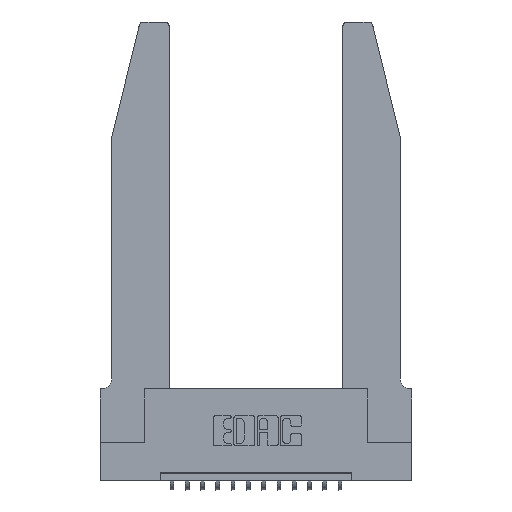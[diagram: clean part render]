
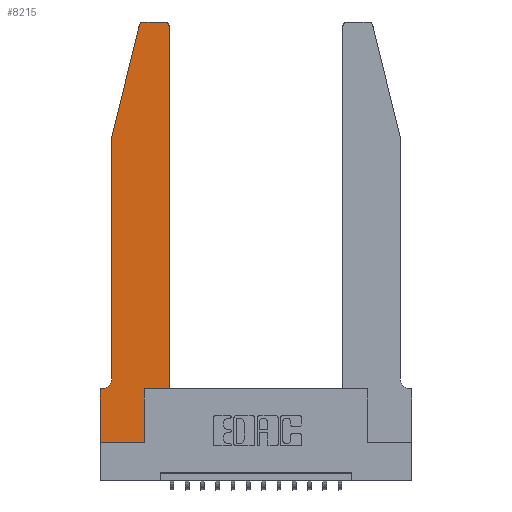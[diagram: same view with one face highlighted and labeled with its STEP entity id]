
A CAD part, top view. The second image highlights one B-rep face of the part: STEP entity #8215.
In plain terms, the highlighted planar face has unit normal (0, 0, 1).
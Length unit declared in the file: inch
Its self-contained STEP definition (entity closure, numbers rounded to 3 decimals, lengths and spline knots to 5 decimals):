
#14 = VERTEX_POINT ( 'NONE', #5899 ) ;
#186 = ORIENTED_EDGE ( 'NONE', *, *, #17065, .T. ) ;
#826 = ORIENTED_EDGE ( 'NONE', *, *, #7847, .T. ) ;
#1065 = CARTESIAN_POINT ( 'NONE',  ( 0.2605, 2.75, 0.37 ) ) ;
#1076 = EDGE_CURVE ( 'NONE', #7995, #10283, #5129, .T. ) ;
#1280 = CIRCLE ( 'NONE', #4419, 0.07 ) ;
#1588 = VERTEX_POINT ( 'NONE', #16901 ) ;
#1635 = EDGE_CURVE ( 'NONE', #1588, #16401, #10755, .T. ) ;
#1659 = VECTOR ( 'NONE', #11710, 39.37008 ) ;
#2126 = CARTESIAN_POINT ( 'NONE',  ( 0., 0., 0.37 ) ) ;
#2230 = CARTESIAN_POINT ( 'NONE',  ( 0.284, 2.72, 0.37 ) ) ;
#2387 = VERTEX_POINT ( 'NONE', #16513 ) ;
#2408 = DIRECTION ( 'NONE',  ( 0., 1., 0. ) ) ;
#2767 = CARTESIAN_POINT ( 'NONE',  ( 0., 0., 0.37 ) ) ;
#3161 = EDGE_CURVE ( 'NONE', #10283, #14, #5533, .T. ) ;
#3262 = VERTEX_POINT ( 'NONE', #2126 ) ;
#3343 = ORIENTED_EDGE ( 'NONE', *, *, #13811, .T. ) ;
#3395 = VECTOR ( 'NONE', #5492, 39.37008 ) ;
#3405 = ORIENTED_EDGE ( 'NONE', *, *, #16926, .T. ) ;
#3450 = ORIENTED_EDGE ( 'NONE', *, *, #16946, .T. ) ;
#3671 = CARTESIAN_POINT ( 'NONE',  ( 0.2865, 0.35, 0.37 ) ) ;
#3999 = AXIS2_PLACEMENT_3D ( 'NONE', #4732, #17258, #11753 ) ;
#4192 = CARTESIAN_POINT ( 'NONE',  ( 0.25487, 2.72718, 0.37 ) ) ;
#4263 = VECTOR ( 'NONE', #7435, 39.37008 ) ;
#4272 = VERTEX_POINT ( 'NONE', #6718 ) ;
#4382 = ORIENTED_EDGE ( 'NONE', *, *, #3161, .T. ) ;
#4390 = DIRECTION ( 'NONE',  ( 0., -1., 0. ) ) ;
#4419 = AXIS2_PLACEMENT_3D ( 'NONE', #12289, #13267, #4938 ) ;
#4446 = CARTESIAN_POINT ( 'NONE',  ( 0., 0., 0.37 ) ) ;
#4488 = FACE_OUTER_BOUND ( 'NONE', #10776, .T. ) ;
#4732 = CARTESIAN_POINT ( 'NONE',  ( 0.4205, 2.72, 0.37 ) ) ;
#4736 = CARTESIAN_POINT ( 'NONE',  ( 0.0755, 2., 0.37 ) ) ;
#4938 = DIRECTION ( 'NONE',  ( -1., 0., 0. ) ) ;
#5013 = AXIS2_PLACEMENT_3D ( 'NONE', #7494, #8884, #10284 ) ;
#5085 = DIRECTION ( 'NONE',  ( 0., 0., 1. ) ) ;
#5129 = LINE ( 'NONE', #14333, #10101 ) ;
#5200 = LINE ( 'NONE', #4446, #15573 ) ;
#5256 = EDGE_CURVE ( 'NONE', #12129, #7332, #7608, .T. ) ;
#5405 = CARTESIAN_POINT ( 'NONE',  ( 0., 0.35, 0.37 ) ) ;
#5492 = DIRECTION ( 'NONE',  ( 1., 0., 0. ) ) ;
#5533 = LINE ( 'NONE', #17791, #8347 ) ;
#5899 = CARTESIAN_POINT ( 'NONE',  ( 0.4505, 2.72, 0.37 ) ) ;
#5978 = LINE ( 'NONE', #1065, #13170 ) ;
#6718 = CARTESIAN_POINT ( 'NONE',  ( 0.2865, 0., 0.37 ) ) ;
#7332 = VERTEX_POINT ( 'NONE', #4736 ) ;
#7435 = DIRECTION ( 'NONE',  ( -1., 0., 0. ) ) ;
#7494 = CARTESIAN_POINT ( 'NONE',  ( 0., 0.35, 0.37 ) ) ;
#7582 = DIRECTION ( 'NONE',  ( 1., 0., 0. ) ) ;
#7608 = LINE ( 'NONE', #14395, #14089 ) ;
#7847 = EDGE_CURVE ( 'NONE', #7332, #11194, #17225, .T. ) ;
#7856 = DIRECTION ( 'NONE',  ( 1., 0., 0. ) ) ;
#7995 = VERTEX_POINT ( 'NONE', #16257 ) ;
#8129 = LINE ( 'NONE', #3671, #8779 ) ;
#8215 = ADVANCED_FACE ( 'NONE', ( #4488 ), #15583, .T. ) ;
#8347 = VECTOR ( 'NONE', #2408, 39.37008 ) ;
#8361 = CIRCLE ( 'NONE', #3999, 0.03 ) ;
#8779 = VECTOR ( 'NONE', #13556, 39.37008 ) ;
#8884 = DIRECTION ( 'NONE',  ( 0., 0., 1. ) ) ;
#8966 = DIRECTION ( 'NONE',  ( -0.239, -0.971, 0. ) ) ;
#9866 = EDGE_CURVE ( 'NONE', #14, #13092, #8361, .T. ) ;
#10101 = VECTOR ( 'NONE', #7582, 39.37008 ) ;
#10283 = VERTEX_POINT ( 'NONE', #16583 ) ;
#10284 = DIRECTION ( 'NONE',  ( 1., 0., 0. ) ) ;
#10676 = EDGE_CURVE ( 'NONE', #4272, #7995, #8129, .T. ) ;
#10755 = LINE ( 'NONE', #11514, #4263 ) ;
#10776 = EDGE_LOOP ( 'NONE', ( #3405, #3450, #16666, #826, #16829, #14975, #3343, #186, #14225, #11814, #4382, #16773 ) ) ;
#11194 = VERTEX_POINT ( 'NONE', #15000 ) ;
#11464 = CARTESIAN_POINT ( 'NONE',  ( 0.0755, 2., 0.37 ) ) ;
#11514 = CARTESIAN_POINT ( 'NONE',  ( 0.0755, 0.35, 0.37 ) ) ;
#11710 = DIRECTION ( 'NONE',  ( 0., -1., 0. ) ) ;
#11753 = DIRECTION ( 'NONE',  ( 1., 0., 0. ) ) ;
#11814 = ORIENTED_EDGE ( 'NONE', *, *, #1076, .T. ) ;
#12076 = CIRCLE ( 'NONE', #13273, 0.03 ) ;
#12129 = VERTEX_POINT ( 'NONE', #4192 ) ;
#12177 = DIRECTION ( 'NONE',  ( -1., 0., 0. ) ) ;
#12289 = CARTESIAN_POINT ( 'NONE',  ( 0.0055, 0.42, 0.37 ) ) ;
#12941 = LINE ( 'NONE', #2767, #3395 ) ;
#13092 = VERTEX_POINT ( 'NONE', #14777 ) ;
#13170 = VECTOR ( 'NONE', #12177, 39.37008 ) ;
#13267 = DIRECTION ( 'NONE',  ( 0., 0., -1. ) ) ;
#13273 = AXIS2_PLACEMENT_3D ( 'NONE', #2230, #5085, #7856 ) ;
#13556 = DIRECTION ( 'NONE',  ( 0., 1., 0. ) ) ;
#13811 = EDGE_CURVE ( 'NONE', #16401, #3262, #5200, .T. ) ;
#14089 = VECTOR ( 'NONE', #8966, 39.37008 ) ;
#14225 = ORIENTED_EDGE ( 'NONE', *, *, #10676, .T. ) ;
#14333 = CARTESIAN_POINT ( 'NONE',  ( 0.4505, 0.35, 0.37 ) ) ;
#14395 = CARTESIAN_POINT ( 'NONE',  ( 0.0755, 2., 0.37 ) ) ;
#14777 = CARTESIAN_POINT ( 'NONE',  ( 0.4205, 2.75, 0.37 ) ) ;
#14975 = ORIENTED_EDGE ( 'NONE', *, *, #1635, .T. ) ;
#15000 = CARTESIAN_POINT ( 'NONE',  ( 0.0755, 0.42, 0.37 ) ) ;
#15573 = VECTOR ( 'NONE', #4390, 39.37008 ) ;
#15583 = PLANE ( 'NONE',  #5013 ) ;
#15698 = EDGE_CURVE ( 'NONE', #11194, #1588, #1280, .T. ) ;
#16257 = CARTESIAN_POINT ( 'NONE',  ( 0.2865, 0.35, 0.37 ) ) ;
#16401 = VERTEX_POINT ( 'NONE', #5405 ) ;
#16513 = CARTESIAN_POINT ( 'NONE',  ( 0.284, 2.75, 0.37 ) ) ;
#16583 = CARTESIAN_POINT ( 'NONE',  ( 0.4505, 0.35, 0.37 ) ) ;
#16666 = ORIENTED_EDGE ( 'NONE', *, *, #5256, .T. ) ;
#16773 = ORIENTED_EDGE ( 'NONE', *, *, #9866, .T. ) ;
#16829 = ORIENTED_EDGE ( 'NONE', *, *, #15698, .T. ) ;
#16901 = CARTESIAN_POINT ( 'NONE',  ( 0.0055, 0.35, 0.37 ) ) ;
#16926 = EDGE_CURVE ( 'NONE', #13092, #2387, #5978, .T. ) ;
#16946 = EDGE_CURVE ( 'NONE', #2387, #12129, #12076, .T. ) ;
#17065 = EDGE_CURVE ( 'NONE', #3262, #4272, #12941, .T. ) ;
#17225 = LINE ( 'NONE', #11464, #1659 ) ;
#17258 = DIRECTION ( 'NONE',  ( 0., 0., 1. ) ) ;
#17791 = CARTESIAN_POINT ( 'NONE',  ( 0.4505, 0.35, 0.37 ) ) ;
